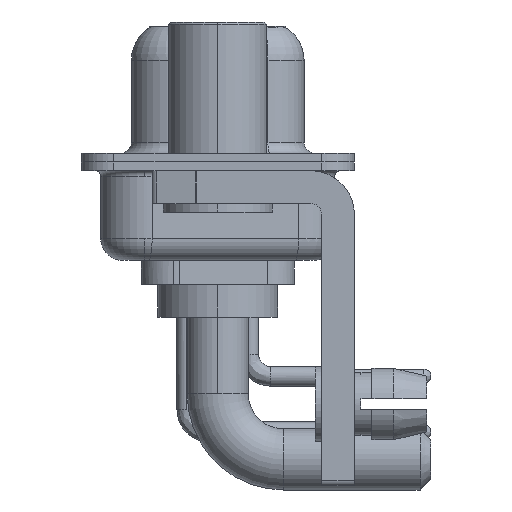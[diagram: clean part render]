
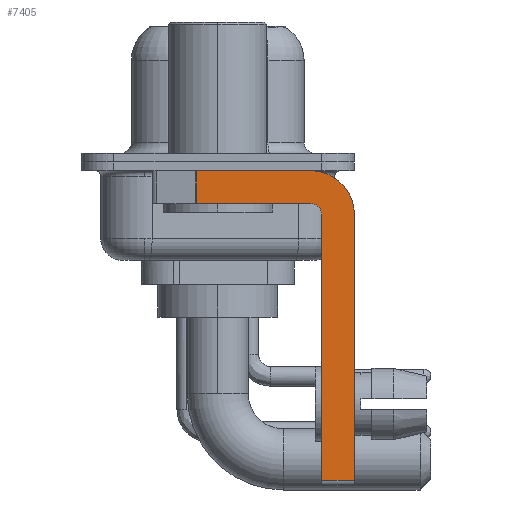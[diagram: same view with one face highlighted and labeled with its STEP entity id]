
A CAD part, left-side view. The second image highlights one B-rep face of the part: STEP entity #7405.
In plain terms, the highlighted planar face has unit normal (-1, 0, 0).
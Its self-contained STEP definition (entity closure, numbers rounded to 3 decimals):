
#132 = VECTOR ( 'NONE', #13288, 1000. ) ;
#568 = VERTEX_POINT ( 'NONE', #24683 ) ;
#1294 = DIRECTION ( 'NONE',  ( 0., 0., -1. ) ) ;
#1551 = EDGE_CURVE ( 'NONE', #3299, #14692, #5726, .T. ) ;
#1568 = LINE ( 'NONE', #23380, #22236 ) ;
#2045 = VECTOR ( 'NONE', #22763, 1000. ) ;
#2177 = CARTESIAN_POINT ( 'NONE',  ( -2.9, -4.25, -1.9 ) ) ;
#2259 = ORIENTED_EDGE ( 'NONE', *, *, #20416, .T. ) ;
#3299 = VERTEX_POINT ( 'NONE', #6806 ) ;
#3886 = CARTESIAN_POINT ( 'NONE',  ( -2.9, -4.25, -2.4 ) ) ;
#4650 = DIRECTION ( 'NONE',  ( 0., 0., -1. ) ) ;
#4790 = CARTESIAN_POINT ( 'NONE',  ( -2.9, -4.25, -2.4 ) ) ;
#4826 = AXIS2_PLACEMENT_3D ( 'NONE', #18863, #5242, #21163 ) ;
#4982 = ORIENTED_EDGE ( 'NONE', *, *, #22268, .F. ) ;
#5242 = DIRECTION ( 'NONE',  ( -1., 0., 0. ) ) ;
#5476 = FACE_OUTER_BOUND ( 'NONE', #8162, .T. ) ;
#5511 = AXIS2_PLACEMENT_3D ( 'NONE', #3886, #27708, #18816 ) ;
#5540 = VECTOR ( 'NONE', #15946, 1000. ) ;
#5546 = VERTEX_POINT ( 'NONE', #18256 ) ;
#5726 = CIRCLE ( 'NONE', #4826, 0.5 ) ;
#6064 = CARTESIAN_POINT ( 'NONE',  ( -2.9, -6.25, -2.4 ) ) ;
#6806 = CARTESIAN_POINT ( 'NONE',  ( -2.9, -4.75, -2.4 ) ) ;
#7199 = CARTESIAN_POINT ( 'NONE',  ( -2.9, -4.25, -14.55 ) ) ;
#7405 = ADVANCED_FACE ( 'NONE', ( #5476 ), #7638, .F. ) ;
#7638 = PLANE ( 'NONE',  #5511 ) ;
#7957 = VERTEX_POINT ( 'NONE', #6064 ) ;
#8162 = EDGE_LOOP ( 'NONE', ( #19300, #2259, #18264, #24343, #4982, #12988, #11447, #23167 ) ) ;
#8458 = CIRCLE ( 'NONE', #26793, 2. ) ;
#9103 = DIRECTION ( 'NONE',  ( 1., 0., 0. ) ) ;
#9362 = LINE ( 'NONE', #7199, #5540 ) ;
#10287 = CARTESIAN_POINT ( 'NONE',  ( -2.9, -4.25, -0.4 ) ) ;
#10603 = CARTESIAN_POINT ( 'NONE',  ( -2.9, 0.978, -1.9 ) ) ;
#10756 = EDGE_CURVE ( 'NONE', #20304, #7957, #8458, .T. ) ;
#11141 = CARTESIAN_POINT ( 'NONE',  ( -2.9, 0.978, -1.9 ) ) ;
#11388 = VERTEX_POINT ( 'NONE', #10603 ) ;
#11447 = ORIENTED_EDGE ( 'NONE', *, *, #12133, .F. ) ;
#11482 = CARTESIAN_POINT ( 'NONE',  ( -2.9, -4.25, -1.9 ) ) ;
#11671 = VECTOR ( 'NONE', #22286, 1000. ) ;
#12133 = EDGE_CURVE ( 'NONE', #7957, #5546, #1568, .T. ) ;
#12519 = LINE ( 'NONE', #2177, #13892 ) ;
#12988 = ORIENTED_EDGE ( 'NONE', *, *, #18754, .T. ) ;
#13288 = DIRECTION ( 'NONE',  ( 0., 0., -1. ) ) ;
#13892 = VECTOR ( 'NONE', #17527, 1000. ) ;
#14692 = VERTEX_POINT ( 'NONE', #11482 ) ;
#15946 = DIRECTION ( 'NONE',  ( 0., -1., 0. ) ) ;
#17527 = DIRECTION ( 'NONE',  ( 0., 1., 0. ) ) ;
#18256 = CARTESIAN_POINT ( 'NONE',  ( -2.9, -6.25, -14.55 ) ) ;
#18264 = ORIENTED_EDGE ( 'NONE', *, *, #25081, .F. ) ;
#18754 = EDGE_CURVE ( 'NONE', #20899, #5546, #9362, .T. ) ;
#18816 = DIRECTION ( 'NONE',  ( 0., 0., -1. ) ) ;
#18863 = CARTESIAN_POINT ( 'NONE',  ( -2.9, -4.25, -2.4 ) ) ;
#19300 = ORIENTED_EDGE ( 'NONE', *, *, #27684, .F. ) ;
#19566 = LINE ( 'NONE', #20135, #11671 ) ;
#20135 = CARTESIAN_POINT ( 'NONE',  ( -2.9, -4.75, -14.8 ) ) ;
#20304 = VERTEX_POINT ( 'NONE', #10287 ) ;
#20416 = EDGE_CURVE ( 'NONE', #568, #11388, #26624, .T. ) ;
#20755 = LINE ( 'NONE', #24916, #2045 ) ;
#20899 = VERTEX_POINT ( 'NONE', #21154 ) ;
#21154 = CARTESIAN_POINT ( 'NONE',  ( -2.9, -4.75, -14.55 ) ) ;
#21163 = DIRECTION ( 'NONE',  ( 0., 0., 1. ) ) ;
#22236 = VECTOR ( 'NONE', #1294, 1000. ) ;
#22268 = EDGE_CURVE ( 'NONE', #20899, #3299, #19566, .T. ) ;
#22286 = DIRECTION ( 'NONE',  ( 0., 0., 1. ) ) ;
#22763 = DIRECTION ( 'NONE',  ( 0., -1., 0. ) ) ;
#23167 = ORIENTED_EDGE ( 'NONE', *, *, #10756, .F. ) ;
#23380 = CARTESIAN_POINT ( 'NONE',  ( -2.9, -6.25, -2.4 ) ) ;
#24343 = ORIENTED_EDGE ( 'NONE', *, *, #1551, .F. ) ;
#24683 = CARTESIAN_POINT ( 'NONE',  ( -2.9, 0.978, -0.4 ) ) ;
#24916 = CARTESIAN_POINT ( 'NONE',  ( -2.9, 3., -0.4 ) ) ;
#25081 = EDGE_CURVE ( 'NONE', #14692, #11388, #12519, .T. ) ;
#26624 = LINE ( 'NONE', #11141, #132 ) ;
#26793 = AXIS2_PLACEMENT_3D ( 'NONE', #4790, #9103, #4650 ) ;
#27684 = EDGE_CURVE ( 'NONE', #568, #20304, #20755, .T. ) ;
#27708 = DIRECTION ( 'NONE',  ( 1., 0., 0. ) ) ;
